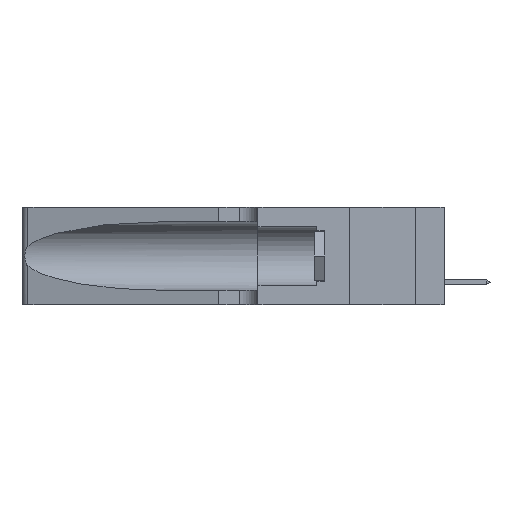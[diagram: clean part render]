
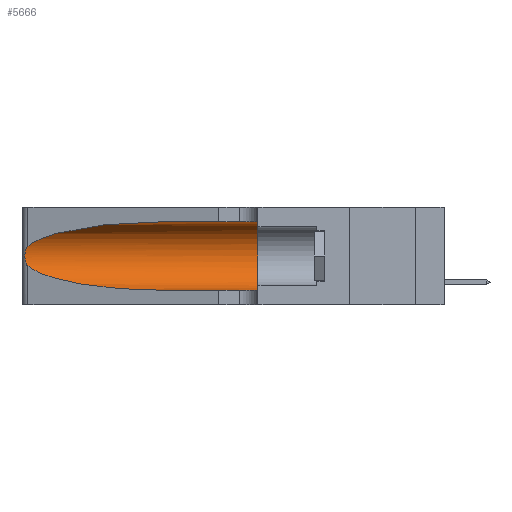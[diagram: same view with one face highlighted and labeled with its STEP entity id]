
A CAD part, left-side view. The second image highlights one B-rep face of the part: STEP entity #5666.
In plain terms, the highlighted cylindrical face has radius 3.308 mm (diameter 6.617 mm), a partial arc.
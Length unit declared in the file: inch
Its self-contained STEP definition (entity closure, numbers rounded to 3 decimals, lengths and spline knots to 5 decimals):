
#115 = VECTOR ( 'NONE', #7835, 39.37008 ) ;
#606 = CARTESIAN_POINT ( 'NONE',  ( 0.2373, 1.15595, 0.28018 ) ) ;
#638 = CARTESIAN_POINT ( 'NONE',  ( 0.26075, 1.23896, 0.178 ) ) ;
#852 = CARTESIAN_POINT ( 'NONE',  ( 0.25555, 1.22993, 0.14849 ) ) ;
#1791 = CYLINDRICAL_SURFACE ( 'NONE', #28656, 0.13025 ) ;
#2633 = ORIENTED_EDGE ( 'NONE', *, *, #12667, .T. ) ;
#2941 = DIRECTION ( 'NONE',  ( 0., -1., 0. ) ) ;
#3019 = CARTESIAN_POINT ( 'NONE',  ( 0.25639, 1.23186, 0.15144 ) ) ;
#3056 = CARTESIAN_POINT ( 'NONE',  ( 0.1305, 1.61858, 0.05475 ) ) ;
#3224 = CARTESIAN_POINT ( 'NONE',  ( 0.25555, 1.22994, 0.2215 ) ) ;
#4318 = VERTEX_POINT ( 'NONE', #19682 ) ;
#4655 = CARTESIAN_POINT ( 'NONE',  ( 0.18966, 0.96281, 0.05475 ) ) ;
#5186 = CARTESIAN_POINT ( 'NONE',  ( 0.1305, 0.35, 0.185 ) ) ;
#5666 = ADVANCED_FACE ( 'NONE', ( #10334 ), #1791, .F. ) ;
#6549 = VERTEX_POINT ( 'NONE', #28218 ) ;
#7170 = CARTESIAN_POINT ( 'NONE',  ( 0.1305, 0.72297, 0.05475 ) ) ;
#7592 = CARTESIAN_POINT ( 'NONE',  ( 0.26075, 1.23896, 0.19203 ) ) ;
#7835 = DIRECTION ( 'NONE',  ( 0., -1., 0. ) ) ;
#8018 = CARTESIAN_POINT ( 'NONE',  ( 0.25787, 1.23484, 0.2124 ) ) ;
#8081 = CARTESIAN_POINT ( 'NONE',  ( 0.1305, 1.61858, 0.185 ) ) ;
#9060 = CARTESIAN_POINT ( 'NONE',  ( 0.1305, 0.72297, 0.31525 ) ) ;
#9596 = LINE ( 'NONE', #29140, #15953 ) ;
#10092 = CARTESIAN_POINT ( 'NONE',  ( 0.25856, 1.23593, 0.16098 ) ) ;
#10301 = CARTESIAN_POINT ( 'NONE',  ( 0.25789, 1.23486, 0.15765 ) ) ;
#10334 = FACE_OUTER_BOUND ( 'NONE', #26934, .T. ) ;
#10485 = ORIENTED_EDGE ( 'NONE', *, *, #17454, .T. ) ;
#10552 = EDGE_CURVE ( 'NONE', #24409, #6549, #9596, .T. ) ;
#11014 =( BOUNDED_CURVE ( )  B_SPLINE_CURVE ( 3, ( #14859, #12387, #606, #29066 ),
 .UNSPECIFIED., .F., .T. ) 
 B_SPLINE_CURVE_WITH_KNOTS ( ( 4, 4 ),
 ( 1.5708, 2.84003 ),
 .UNSPECIFIED. ) 
 CURVE ( )  GEOMETRIC_REPRESENTATION_ITEM ( )  RATIONAL_B_SPLINE_CURVE ( ( 1., 0.87, 0.87, 1. ) ) 
 REPRESENTATION_ITEM ( '' )  );
#12387 = CARTESIAN_POINT ( 'NONE',  ( 0.18966, 0.96281, 0.31525 ) ) ;
#12530 = CARTESIAN_POINT ( 'NONE',  ( 0.1305, 0.72297, 0.05475 ) ) ;
#12667 = EDGE_CURVE ( 'NONE', #24409, #19305, #11014, .T. ) ;
#13116 = DIRECTION ( 'NONE',  ( 0., 0., -1. ) ) ;
#14041 = ORIENTED_EDGE ( 'NONE', *, *, #30379, .T. ) ;
#14521 = VERTEX_POINT ( 'NONE', #12530 ) ;
#14859 = CARTESIAN_POINT ( 'NONE',  ( 0.1305, 0.72297, 0.31525 ) ) ;
#15187 = B_SPLINE_CURVE_WITH_KNOTS ( 'NONE', 3,
 ( #24381, #3224, #27015, #8018, #19922, #17311, #7592, #638, #24270, #10092, #10301, #3019, #852, #19713 ),
 .UNSPECIFIED., .F., .F.,
 ( 4, 2, 2, 2, 2, 2, 4 ),
 ( 0., 0.00027, 0.00053, 0.00107, 0.0016, 0.00187, 0.00214 ),
 .UNSPECIFIED. ) ;
#15237 = AXIS2_PLACEMENT_3D ( 'NONE', #5186, #26389, #21992 ) ;
#15953 = VECTOR ( 'NONE', #2941, 39.37008 ) ;
#16980 = EDGE_CURVE ( 'NONE', #19305, #20880, #15187, .T. ) ;
#17311 = CARTESIAN_POINT ( 'NONE',  ( 0.26018, 1.23835, 0.19895 ) ) ;
#17454 = EDGE_CURVE ( 'NONE', #14521, #4318, #27384, .T. ) ;
#17602 = DIRECTION ( 'NONE',  ( 0., -1., 0. ) ) ;
#19305 = VERTEX_POINT ( 'NONE', #24172 ) ;
#19407 =( BOUNDED_CURVE ( )  B_SPLINE_CURVE ( 3, ( #20580, #25354, #4655, #7170 ),
 .UNSPECIFIED., .F., .F. ) 
 B_SPLINE_CURVE_WITH_KNOTS ( ( 4, 4 ),
 ( 3.44316, 4.71239 ),
 .UNSPECIFIED. ) 
 CURVE ( )  GEOMETRIC_REPRESENTATION_ITEM ( )  RATIONAL_B_SPLINE_CURVE ( ( 1., 0.87, 0.87, 1. ) ) 
 REPRESENTATION_ITEM ( '' )  );
#19682 = CARTESIAN_POINT ( 'NONE',  ( 0.1305, 0.35, 0.05475 ) ) ;
#19713 = CARTESIAN_POINT ( 'NONE',  ( 0.25487, 1.22718, 0.14631 ) ) ;
#19922 = CARTESIAN_POINT ( 'NONE',  ( 0.25854, 1.2359, 0.20912 ) ) ;
#20580 = CARTESIAN_POINT ( 'NONE',  ( 0.25487, 1.22718, 0.14631 ) ) ;
#20712 = ORIENTED_EDGE ( 'NONE', *, *, #24007, .F. ) ;
#20864 = CARTESIAN_POINT ( 'NONE',  ( 0.25487, 1.22718, 0.14631 ) ) ;
#20880 = VERTEX_POINT ( 'NONE', #20864 ) ;
#21992 = DIRECTION ( 'NONE',  ( 0., 0., 1. ) ) ;
#24007 = EDGE_CURVE ( 'NONE', #6549, #4318, #26651, .T. ) ;
#24172 = CARTESIAN_POINT ( 'NONE',  ( 0.25487, 1.22718, 0.22369 ) ) ;
#24270 = CARTESIAN_POINT ( 'NONE',  ( 0.26017, 1.23833, 0.17102 ) ) ;
#24381 = CARTESIAN_POINT ( 'NONE',  ( 0.25487, 1.22718, 0.22369 ) ) ;
#24409 = VERTEX_POINT ( 'NONE', #9060 ) ;
#25354 = CARTESIAN_POINT ( 'NONE',  ( 0.2373, 1.15595, 0.08982 ) ) ;
#26389 = DIRECTION ( 'NONE',  ( 0., 1., 0. ) ) ;
#26651 = CIRCLE ( 'NONE', #15237, 0.13025 ) ;
#26934 = EDGE_LOOP ( 'NONE', ( #2633, #28586, #14041, #10485, #20712, #30636 ) ) ;
#27015 = CARTESIAN_POINT ( 'NONE',  ( 0.25639, 1.23184, 0.21858 ) ) ;
#27384 = LINE ( 'NONE', #3056, #115 ) ;
#28218 = CARTESIAN_POINT ( 'NONE',  ( 0.1305, 0.35, 0.31525 ) ) ;
#28586 = ORIENTED_EDGE ( 'NONE', *, *, #16980, .T. ) ;
#28656 = AXIS2_PLACEMENT_3D ( 'NONE', #8081, #17602, #13116 ) ;
#29066 = CARTESIAN_POINT ( 'NONE',  ( 0.25487, 1.22718, 0.22369 ) ) ;
#29140 = CARTESIAN_POINT ( 'NONE',  ( 0.1305, 1.61858, 0.31525 ) ) ;
#30379 = EDGE_CURVE ( 'NONE', #20880, #14521, #19407, .T. ) ;
#30636 = ORIENTED_EDGE ( 'NONE', *, *, #10552, .F. ) ;
